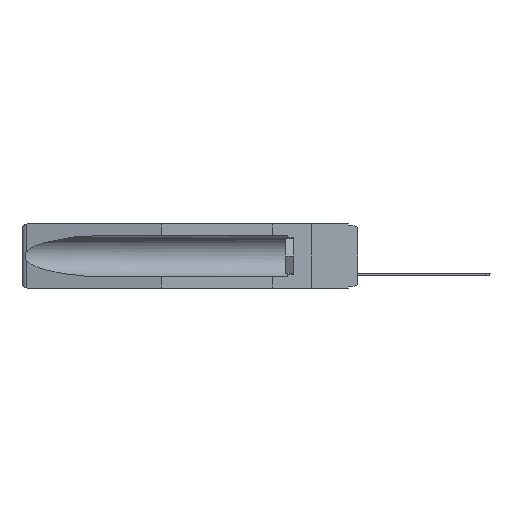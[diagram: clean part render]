
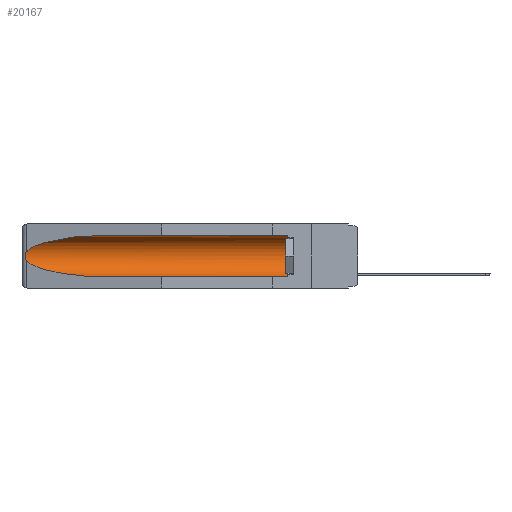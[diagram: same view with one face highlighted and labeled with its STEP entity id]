
A CAD part, left-side view. The second image highlights one B-rep face of the part: STEP entity #20167.
In plain terms, the highlighted cylindrical face has radius 2.857 mm (diameter 5.715 mm), a partial arc.
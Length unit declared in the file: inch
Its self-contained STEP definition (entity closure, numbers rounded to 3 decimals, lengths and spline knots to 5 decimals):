
#243 = CARTESIAN_POINT ( 'NONE',  ( 0.2675, 1.53308, -0.17534 ) ) ;
#336 = ORIENTED_EDGE ( 'NONE', *, *, #17589, .T. ) ;
#1078 = ORIENTED_EDGE ( 'NONE', *, *, #10172, .T. ) ;
#1675 = VERTEX_POINT ( 'NONE', #11149 ) ;
#1727 = CIRCLE ( 'NONE', #17258, 0.1125 ) ;
#2096 = CARTESIAN_POINT ( 'NONE',  ( 0.26597, 1.52961, -0.15275 ) ) ;
#2164 = CARTESIAN_POINT ( 'NONE',  ( 0.26537, 1.52718, -0.19328 ) ) ;
#2260 = CARTESIAN_POINT ( 'NONE',  ( 0.155, 1.07973, -0.284 ) ) ;
#2908 = CARTESIAN_POINT ( 'NONE',  ( 0.21114, 1.30732, -0.059 ) ) ;
#3316 = CARTESIAN_POINT ( 'NONE',  ( 0.26537, 1.52718, -0.19328 ) ) ;
#3656 = CARTESIAN_POINT ( 'NONE',  ( 0.155, 0.126, -0.1715 ) ) ;
#3759 = CARTESIAN_POINT ( 'NONE',  ( 0.155, 1.07973, -0.284 ) ) ;
#4069 = CARTESIAN_POINT ( 'NONE',  ( 0.2673, 1.5327, -0.16383 ) ) ;
#4156 = CARTESIAN_POINT ( 'NONE',  ( 0.21114, 1.30732, -0.284 ) ) ;
#4159 = CARTESIAN_POINT ( 'NONE',  ( 0.2675, 1.53308, -0.16763 ) ) ;
#4697 = CARTESIAN_POINT ( 'NONE',  ( 0.26537, 1.52718, -0.14972 ) ) ;
#6015 = CARTESIAN_POINT ( 'NONE',  ( 0.26655, 1.53094, -0.18657 ) ) ;
#6063 = CARTESIAN_POINT ( 'NONE',  ( 0.155, 1.07973, -0.059 ) ) ;
#6654 = EDGE_CURVE ( 'NONE', #21831, #24913, #7857, .T. ) ;
#7012 = DIRECTION ( 'NONE',  ( 0., 0., 1. ) ) ;
#7383 = B_SPLINE_CURVE_WITH_KNOTS ( 'NONE', 3,
 ( #19532, #2096, #11761, #4069, #4159, #243, #23559, #6015, #19630, #8222 ),
 .UNSPECIFIED., .F., .F.,
 ( 4, 2, 2, 2, 4 ),
 ( 0., 0.00029, 0.00058, 0.00087, 0.00117 ),
 .UNSPECIFIED. ) ;
#7564 = CARTESIAN_POINT ( 'NONE',  ( 0.155, 0.126, -0.284 ) ) ;
#7857 =( BOUNDED_CURVE ( )  B_SPLINE_CURVE ( 3, ( #2164, #15897, #4156, #2260 ),
 .UNSPECIFIED., .F., .F. ) 
 B_SPLINE_CURVE_WITH_KNOTS ( ( 4, 4 ),
 ( 0.1948, 1.5708 ),
 .UNSPECIFIED. ) 
 CURVE ( )  GEOMETRIC_REPRESENTATION_ITEM ( )  RATIONAL_B_SPLINE_CURVE ( ( 1., 0.848, 0.848, 1. ) ) 
 REPRESENTATION_ITEM ( '' )  );
#8222 = CARTESIAN_POINT ( 'NONE',  ( 0.26537, 1.52718, -0.19328 ) ) ;
#8573 = ORIENTED_EDGE ( 'NONE', *, *, #10511, .T. ) ;
#8606 = EDGE_LOOP ( 'NONE', ( #336, #23463, #12538, #17476, #8573, #1078 ) ) ;
#9533 = VERTEX_POINT ( 'NONE', #6063 ) ;
#10172 = EDGE_CURVE ( 'NONE', #11766, #9533, #19394, .T. ) ;
#10511 = EDGE_CURVE ( 'NONE', #13466, #11766, #1727, .T. ) ;
#11149 = CARTESIAN_POINT ( 'NONE',  ( 0.26537, 1.52718, -0.14972 ) ) ;
#11180 = DIRECTION ( 'NONE',  ( 0., -1., 0. ) ) ;
#11249 = DIRECTION ( 'NONE',  ( 0., 1., 0. ) ) ;
#11761 = CARTESIAN_POINT ( 'NONE',  ( 0.26654, 1.53092, -0.15636 ) ) ;
#11766 = VERTEX_POINT ( 'NONE', #13399 ) ;
#12538 = ORIENTED_EDGE ( 'NONE', *, *, #6654, .T. ) ;
#13212 = DIRECTION ( 'NONE',  ( 0., 0., 1. ) ) ;
#13399 = CARTESIAN_POINT ( 'NONE',  ( 0.155, 0.126, -0.059 ) ) ;
#13466 = VERTEX_POINT ( 'NONE', #7564 ) ;
#14246 = VECTOR ( 'NONE', #11249, 39.37008 ) ;
#14296 = FACE_OUTER_BOUND ( 'NONE', #8606, .T. ) ;
#15897 = CARTESIAN_POINT ( 'NONE',  ( 0.25451, 1.48313, -0.24835 ) ) ;
#16079 = EDGE_CURVE ( 'NONE', #1675, #21831, #7383, .T. ) ;
#16471 =( BOUNDED_CURVE ( )  B_SPLINE_CURVE ( 3, ( #18156, #2908, #22212, #4697 ),
 .UNSPECIFIED., .F., .F. ) 
 B_SPLINE_CURVE_WITH_KNOTS ( ( 4, 4 ),
 ( 4.71239, 6.08839 ),
 .UNSPECIFIED. ) 
 CURVE ( )  GEOMETRIC_REPRESENTATION_ITEM ( )  RATIONAL_B_SPLINE_CURVE ( ( 1., 0.848, 0.848, 1. ) ) 
 REPRESENTATION_ITEM ( '' )  );
#16593 = DIRECTION ( 'NONE',  ( 0., 1., 0. ) ) ;
#17090 = CARTESIAN_POINT ( 'NONE',  ( 0.155, -0.30754, -0.059 ) ) ;
#17258 = AXIS2_PLACEMENT_3D ( 'NONE', #3656, #11180, #13212 ) ;
#17476 = ORIENTED_EDGE ( 'NONE', *, *, #24390, .F. ) ;
#17589 = EDGE_CURVE ( 'NONE', #9533, #1675, #16471, .T. ) ;
#17783 = VECTOR ( 'NONE', #21297, 39.37008 ) ;
#18156 = CARTESIAN_POINT ( 'NONE',  ( 0.155, 1.07973, -0.059 ) ) ;
#18769 = CARTESIAN_POINT ( 'NONE',  ( 0.155, -0.30754, -0.1715 ) ) ;
#19394 = LINE ( 'NONE', #17090, #14246 ) ;
#19532 = CARTESIAN_POINT ( 'NONE',  ( 0.26537, 1.52718, -0.14972 ) ) ;
#19630 = CARTESIAN_POINT ( 'NONE',  ( 0.26597, 1.5296, -0.19026 ) ) ;
#20167 = ADVANCED_FACE ( 'NONE', ( #14296 ), #24912, .F. ) ;
#20462 = AXIS2_PLACEMENT_3D ( 'NONE', #18769, #16593, #7012 ) ;
#21297 = DIRECTION ( 'NONE',  ( 0., 1., 0. ) ) ;
#21831 = VERTEX_POINT ( 'NONE', #3316 ) ;
#22212 = CARTESIAN_POINT ( 'NONE',  ( 0.25451, 1.48313, -0.09465 ) ) ;
#23463 = ORIENTED_EDGE ( 'NONE', *, *, #16079, .T. ) ;
#23523 = CARTESIAN_POINT ( 'NONE',  ( 0.155, -0.30754, -0.284 ) ) ;
#23559 = CARTESIAN_POINT ( 'NONE',  ( 0.2673, 1.53269, -0.17917 ) ) ;
#24390 = EDGE_CURVE ( 'NONE', #13466, #24913, #24804, .T. ) ;
#24804 = LINE ( 'NONE', #23523, #17783 ) ;
#24912 = CYLINDRICAL_SURFACE ( 'NONE', #20462, 0.1125 ) ;
#24913 = VERTEX_POINT ( 'NONE', #3759 ) ;
